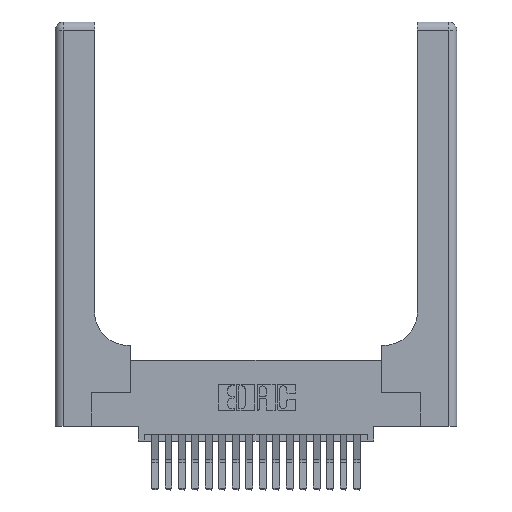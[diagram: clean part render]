
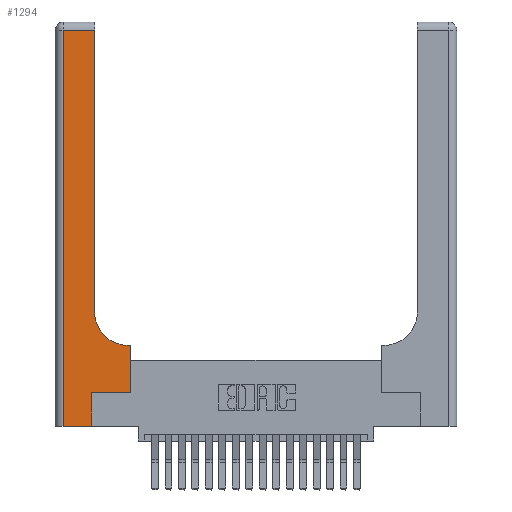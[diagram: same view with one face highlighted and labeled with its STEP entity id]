
A CAD part, top view. The second image highlights one B-rep face of the part: STEP entity #1294.
In plain terms, the highlighted planar face has unit normal (0, 0, 1).
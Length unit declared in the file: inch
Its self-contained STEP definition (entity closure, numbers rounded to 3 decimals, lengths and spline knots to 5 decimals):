
#2 = ORIENTED_EDGE ( 'NONE', *, *, #15527, .T. ) ;
#67 = EDGE_CURVE ( 'NONE', #9709, #5384, #12228, .T. ) ;
#453 = DIRECTION ( 'NONE',  ( 0., 1., 0. ) ) ;
#485 = VERTEX_POINT ( 'NONE', #7059 ) ;
#605 = PLANE ( 'NONE',  #18078 ) ;
#647 = EDGE_CURVE ( 'NONE', #15333, #18356, #13498, .T. ) ;
#784 = ORIENTED_EDGE ( 'NONE', *, *, #8142, .T. ) ;
#928 = LINE ( 'NONE', #5399, #8958 ) ;
#1294 = ADVANCED_FACE ( 'NONE', ( #5182 ), #605, .F. ) ;
#1407 = DIRECTION ( 'NONE',  ( -1., 0., 0. ) ) ;
#2197 = CARTESIAN_POINT ( 'NONE',  ( 0.5415, 0.6, 0.37 ) ) ;
#2363 = ORIENTED_EDGE ( 'NONE', *, *, #14312, .T. ) ;
#2469 = DIRECTION ( 'NONE',  ( 1., 0., 0. ) ) ;
#2848 = EDGE_CURVE ( 'NONE', #15799, #11877, #6171, .T. ) ;
#4006 = EDGE_CURVE ( 'NONE', #11877, #9709, #14796, .T. ) ;
#5089 = ORIENTED_EDGE ( 'NONE', *, *, #67, .T. ) ;
#5112 = EDGE_CURVE ( 'NONE', #14625, #485, #17909, .T. ) ;
#5182 = FACE_OUTER_BOUND ( 'NONE', #18040, .T. ) ;
#5384 = VERTEX_POINT ( 'NONE', #17732 ) ;
#5399 = CARTESIAN_POINT ( 'NONE',  ( 0.269, 0., 0.37 ) ) ;
#5890 = DIRECTION ( 'NONE',  ( 0., 0., -1. ) ) ;
#6099 = CARTESIAN_POINT ( 'NONE',  ( 0.06, 0., 0.37 ) ) ;
#6171 = CIRCLE ( 'NONE', #9626, 0.25 ) ;
#6337 = ORIENTED_EDGE ( 'NONE', *, *, #15686, .T. ) ;
#6631 = VECTOR ( 'NONE', #10102, 39.37008 ) ;
#6768 = VECTOR ( 'NONE', #9086, 39.37008 ) ;
#7059 = CARTESIAN_POINT ( 'NONE',  ( 0.5585, 0.6, 0.37 ) ) ;
#7136 = VECTOR ( 'NONE', #2469, 39.37008 ) ;
#7338 = CARTESIAN_POINT ( 'NONE',  ( 0.2915, 3., 0.37 ) ) ;
#7550 = VECTOR ( 'NONE', #9478, 39.37008 ) ;
#8142 = EDGE_CURVE ( 'NONE', #18356, #20417, #928, .T. ) ;
#8226 = CARTESIAN_POINT ( 'NONE',  ( 0.269, 0.25, 0.37 ) ) ;
#8421 = CARTESIAN_POINT ( 'NONE',  ( 0., 2.94, 0.37 ) ) ;
#8958 = VECTOR ( 'NONE', #453, 39.37008 ) ;
#9086 = DIRECTION ( 'NONE',  ( 0., 1., 0. ) ) ;
#9230 = DIRECTION ( 'NONE',  ( 1., 0., 0. ) ) ;
#9478 = DIRECTION ( 'NONE',  ( -1., 0., 0. ) ) ;
#9626 = AXIS2_PLACEMENT_3D ( 'NONE', #20877, #17916, #12680 ) ;
#9709 = VERTEX_POINT ( 'NONE', #13013 ) ;
#9784 = CARTESIAN_POINT ( 'NONE',  ( 0.2915, 0.6, 0.37 ) ) ;
#9854 = VECTOR ( 'NONE', #9230, 39.37008 ) ;
#10102 = DIRECTION ( 'NONE',  ( 0., -1., 0. ) ) ;
#10495 = LINE ( 'NONE', #8226, #7136 ) ;
#11235 = CARTESIAN_POINT ( 'NONE',  ( 0., 3., 0.37 ) ) ;
#11455 = CARTESIAN_POINT ( 'NONE',  ( 0.2915, 0.85, 0.37 ) ) ;
#11623 = CARTESIAN_POINT ( 'NONE',  ( 0.06, 3., 0.37 ) ) ;
#11877 = VERTEX_POINT ( 'NONE', #11455 ) ;
#11893 = ORIENTED_EDGE ( 'NONE', *, *, #4006, .T. ) ;
#11894 = CARTESIAN_POINT ( 'NONE',  ( 0.269, 0., 0.37 ) ) ;
#12228 = LINE ( 'NONE', #8421, #7550 ) ;
#12274 = ORIENTED_EDGE ( 'NONE', *, *, #647, .T. ) ;
#12318 = CARTESIAN_POINT ( 'NONE',  ( 0.5585, 0.25, 0.37 ) ) ;
#12680 = DIRECTION ( 'NONE',  ( 1., 0., 0. ) ) ;
#13013 = CARTESIAN_POINT ( 'NONE',  ( 0.2915, 2.94, 0.37 ) ) ;
#13498 = LINE ( 'NONE', #19033, #9854 ) ;
#14312 = EDGE_CURVE ( 'NONE', #485, #15799, #16309, .T. ) ;
#14625 = VERTEX_POINT ( 'NONE', #12318 ) ;
#14658 = DIRECTION ( 'NONE',  ( -1., 0., 0. ) ) ;
#14796 = LINE ( 'NONE', #7338, #6768 ) ;
#15333 = VERTEX_POINT ( 'NONE', #6099 ) ;
#15527 = EDGE_CURVE ( 'NONE', #5384, #15333, #17545, .T. ) ;
#15686 = EDGE_CURVE ( 'NONE', #20417, #14625, #10495, .T. ) ;
#15799 = VERTEX_POINT ( 'NONE', #2197 ) ;
#16309 = LINE ( 'NONE', #9784, #19678 ) ;
#16640 = ORIENTED_EDGE ( 'NONE', *, *, #5112, .T. ) ;
#17545 = LINE ( 'NONE', #11623, #6631 ) ;
#17721 = CARTESIAN_POINT ( 'NONE',  ( 0.269, 0.25, 0.37 ) ) ;
#17732 = CARTESIAN_POINT ( 'NONE',  ( 0.06, 2.94, 0.37 ) ) ;
#17909 = LINE ( 'NONE', #18214, #19474 ) ;
#17916 = DIRECTION ( 'NONE',  ( 0., 0., -1. ) ) ;
#18040 = EDGE_LOOP ( 'NONE', ( #11893, #5089, #2, #12274, #784, #6337, #16640, #2363, #20039 ) ) ;
#18078 = AXIS2_PLACEMENT_3D ( 'NONE', #11235, #5890, #1407 ) ;
#18214 = CARTESIAN_POINT ( 'NONE',  ( 0.5585, 0.25, 0.37 ) ) ;
#18356 = VERTEX_POINT ( 'NONE', #11894 ) ;
#19033 = CARTESIAN_POINT ( 'NONE',  ( 0., 0., 0.37 ) ) ;
#19474 = VECTOR ( 'NONE', #19607, 39.37008 ) ;
#19607 = DIRECTION ( 'NONE',  ( 0., 1., 0. ) ) ;
#19678 = VECTOR ( 'NONE', #14658, 39.37008 ) ;
#20039 = ORIENTED_EDGE ( 'NONE', *, *, #2848, .T. ) ;
#20417 = VERTEX_POINT ( 'NONE', #17721 ) ;
#20877 = CARTESIAN_POINT ( 'NONE',  ( 0.5415, 0.85, 0.37 ) ) ;
